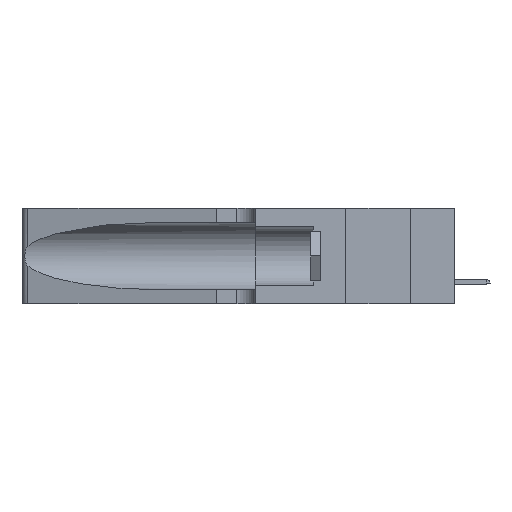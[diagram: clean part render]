
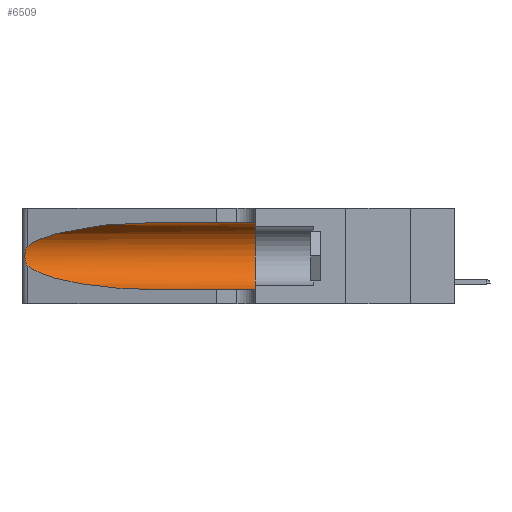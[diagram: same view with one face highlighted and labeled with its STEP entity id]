
A CAD part, left-side view. The second image highlights one B-rep face of the part: STEP entity #6509.
In plain terms, the highlighted cylindrical face has radius 3.308 mm (diameter 6.617 mm), a partial arc.
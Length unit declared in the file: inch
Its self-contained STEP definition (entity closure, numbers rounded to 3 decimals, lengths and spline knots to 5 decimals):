
#66 = ORIENTED_EDGE ( 'NONE', *, *, #324, .F. ) ;
#209 =( BOUNDED_CURVE ( )  B_SPLINE_CURVE ( 3, ( #4250, #5102, #21323, #11147 ),
 .UNSPECIFIED., .F., .F. ) 
 B_SPLINE_CURVE_WITH_KNOTS ( ( 4, 4 ),
 ( 1.5708, 2.84003 ),
 .UNSPECIFIED. ) 
 CURVE ( )  GEOMETRIC_REPRESENTATION_ITEM ( )  RATIONAL_B_SPLINE_CURVE ( ( 1., 0.87, 0.87, 1. ) ) 
 REPRESENTATION_ITEM ( '' )  );
#324 = EDGE_CURVE ( 'NONE', #5755, #2010, #24566, .T. ) ;
#908 = CARTESIAN_POINT ( 'NONE',  ( 0.25487, 1.22718, 0.22369 ) ) ;
#1230 = ORIENTED_EDGE ( 'NONE', *, *, #6104, .T. ) ;
#1646 = CARTESIAN_POINT ( 'NONE',  ( 0.1305, 1.61858, 0.05475 ) ) ;
#2010 = VERTEX_POINT ( 'NONE', #33708 ) ;
#2029 = VERTEX_POINT ( 'NONE', #908 ) ;
#2217 = VECTOR ( 'NONE', #27793, 39.37008 ) ;
#2431 = CYLINDRICAL_SURFACE ( 'NONE', #26626, 0.13025 ) ;
#2580 = CARTESIAN_POINT ( 'NONE',  ( 0.1305, 0.72297, 0.31525 ) ) ;
#2985 = DIRECTION ( 'NONE',  ( 0., 1., 0. ) ) ;
#4221 = CARTESIAN_POINT ( 'NONE',  ( 0.25639, 1.23186, 0.15144 ) ) ;
#4250 = CARTESIAN_POINT ( 'NONE',  ( 0.1305, 0.72297, 0.31525 ) ) ;
#4437 = CARTESIAN_POINT ( 'NONE',  ( 0.25487, 1.22718, 0.14631 ) ) ;
#4827 = VERTEX_POINT ( 'NONE', #8903 ) ;
#5102 = CARTESIAN_POINT ( 'NONE',  ( 0.18966, 0.96281, 0.31525 ) ) ;
#5755 = VERTEX_POINT ( 'NONE', #2580 ) ;
#6104 = EDGE_CURVE ( 'NONE', #4827, #20445, #12067, .T. ) ;
#6509 = ADVANCED_FACE ( 'NONE', ( #18833 ), #2431, .F. ) ;
#6750 = CARTESIAN_POINT ( 'NONE',  ( 0.1305, 0.72297, 0.05475 ) ) ;
#7440 = CARTESIAN_POINT ( 'NONE',  ( 0.25856, 1.23593, 0.16098 ) ) ;
#7654 = CARTESIAN_POINT ( 'NONE',  ( 0.25854, 1.2359, 0.20912 ) ) ;
#7660 = LINE ( 'NONE', #1646, #42577 ) ;
#7767 = EDGE_CURVE ( 'NONE', #20445, #29322, #7660, .T. ) ;
#8114 = CARTESIAN_POINT ( 'NONE',  ( 0.1305, 0.72297, 0.05475 ) ) ;
#8294 = CARTESIAN_POINT ( 'NONE',  ( 0.26018, 1.23835, 0.19895 ) ) ;
#8390 = ORIENTED_EDGE ( 'NONE', *, *, #15445, .T. ) ;
#8903 = CARTESIAN_POINT ( 'NONE',  ( 0.25487, 1.22718, 0.14631 ) ) ;
#9997 = EDGE_CURVE ( 'NONE', #2010, #29322, #27450, .T. ) ;
#10695 = CARTESIAN_POINT ( 'NONE',  ( 0.26075, 1.23896, 0.178 ) ) ;
#11114 = CARTESIAN_POINT ( 'NONE',  ( 0.26075, 1.23896, 0.19203 ) ) ;
#11122 = ORIENTED_EDGE ( 'NONE', *, *, #7767, .T. ) ;
#11147 = CARTESIAN_POINT ( 'NONE',  ( 0.25487, 1.22718, 0.22369 ) ) ;
#11846 = EDGE_CURVE ( 'NONE', #2029, #4827, #11976, .T. ) ;
#11976 = B_SPLINE_CURVE_WITH_KNOTS ( 'NONE', 3,
 ( #20863, #37232, #31217, #37874, #7654, #8294, #11114, #10695, #37024, #7440, #33790, #4221, #34011, #4437 ),
 .UNSPECIFIED., .F., .F.,
 ( 4, 2, 2, 2, 2, 2, 4 ),
 ( 0., 0.00027, 0.00053, 0.00107, 0.0016, 0.00187, 0.00214 ),
 .UNSPECIFIED. ) ;
#12067 =( BOUNDED_CURVE ( )  B_SPLINE_CURVE ( 3, ( #13251, #38918, #29436, #6750 ),
 .UNSPECIFIED., .F., .T. ) 
 B_SPLINE_CURVE_WITH_KNOTS ( ( 4, 4 ),
 ( 3.44316, 4.71239 ),
 .UNSPECIFIED. ) 
 CURVE ( )  GEOMETRIC_REPRESENTATION_ITEM ( )  RATIONAL_B_SPLINE_CURVE ( ( 1., 0.87, 0.87, 1. ) ) 
 REPRESENTATION_ITEM ( '' )  );
#12568 = ORIENTED_EDGE ( 'NONE', *, *, #9997, .F. ) ;
#13224 = ORIENTED_EDGE ( 'NONE', *, *, #11846, .T. ) ;
#13251 = CARTESIAN_POINT ( 'NONE',  ( 0.25487, 1.22718, 0.14631 ) ) ;
#14399 = CARTESIAN_POINT ( 'NONE',  ( 0.1305, 1.61858, 0.31525 ) ) ;
#15445 = EDGE_CURVE ( 'NONE', #5755, #2029, #209, .T. ) ;
#16811 = CARTESIAN_POINT ( 'NONE',  ( 0.1305, 0.35, 0.05475 ) ) ;
#18833 = FACE_OUTER_BOUND ( 'NONE', #22081, .T. ) ;
#20445 = VERTEX_POINT ( 'NONE', #8114 ) ;
#20863 = CARTESIAN_POINT ( 'NONE',  ( 0.25487, 1.22718, 0.22369 ) ) ;
#21323 = CARTESIAN_POINT ( 'NONE',  ( 0.2373, 1.15595, 0.28018 ) ) ;
#22081 = EDGE_LOOP ( 'NONE', ( #8390, #13224, #1230, #11122, #12568, #66 ) ) ;
#22849 = CARTESIAN_POINT ( 'NONE',  ( 0.1305, 0.35, 0.185 ) ) ;
#23313 = AXIS2_PLACEMENT_3D ( 'NONE', #22849, #2985, #23715 ) ;
#23715 = DIRECTION ( 'NONE',  ( 0., 0., 1. ) ) ;
#24566 = LINE ( 'NONE', #14399, #2217 ) ;
#26626 = AXIS2_PLACEMENT_3D ( 'NONE', #37619, #28761, #41059 ) ;
#27349 = DIRECTION ( 'NONE',  ( 0., -1., 0. ) ) ;
#27450 = CIRCLE ( 'NONE', #23313, 0.13025 ) ;
#27793 = DIRECTION ( 'NONE',  ( 0., -1., 0. ) ) ;
#28761 = DIRECTION ( 'NONE',  ( 0., -1., 0. ) ) ;
#29322 = VERTEX_POINT ( 'NONE', #16811 ) ;
#29436 = CARTESIAN_POINT ( 'NONE',  ( 0.18966, 0.96281, 0.05475 ) ) ;
#31217 = CARTESIAN_POINT ( 'NONE',  ( 0.25639, 1.23184, 0.21858 ) ) ;
#33708 = CARTESIAN_POINT ( 'NONE',  ( 0.1305, 0.35, 0.31525 ) ) ;
#33790 = CARTESIAN_POINT ( 'NONE',  ( 0.25789, 1.23486, 0.15765 ) ) ;
#34011 = CARTESIAN_POINT ( 'NONE',  ( 0.25555, 1.22993, 0.14849 ) ) ;
#37024 = CARTESIAN_POINT ( 'NONE',  ( 0.26017, 1.23833, 0.17102 ) ) ;
#37232 = CARTESIAN_POINT ( 'NONE',  ( 0.25555, 1.22994, 0.2215 ) ) ;
#37619 = CARTESIAN_POINT ( 'NONE',  ( 0.1305, 1.61858, 0.185 ) ) ;
#37874 = CARTESIAN_POINT ( 'NONE',  ( 0.25787, 1.23484, 0.2124 ) ) ;
#38918 = CARTESIAN_POINT ( 'NONE',  ( 0.2373, 1.15595, 0.08982 ) ) ;
#41059 = DIRECTION ( 'NONE',  ( 0., 0., -1. ) ) ;
#42577 = VECTOR ( 'NONE', #27349, 39.37008 ) ;
